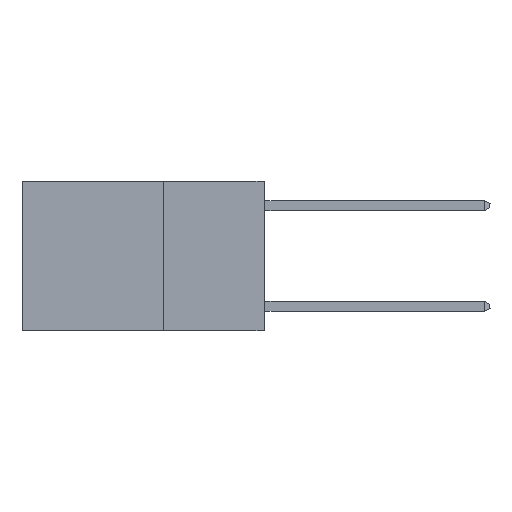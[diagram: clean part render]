
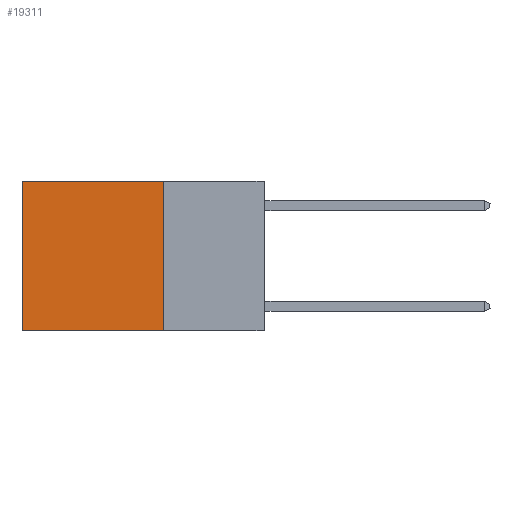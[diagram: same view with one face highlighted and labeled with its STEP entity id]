
A CAD part, left-side view. The second image highlights one B-rep face of the part: STEP entity #19311.
In plain terms, the highlighted planar face has unit normal (-1, 0, 0).
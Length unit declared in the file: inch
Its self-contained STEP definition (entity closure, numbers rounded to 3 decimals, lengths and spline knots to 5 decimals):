
#1014 = LINE ( 'NONE', #16005, #12739 ) ;
#1134 = DIRECTION ( 'NONE',  ( 0., 1., 0. ) ) ;
#2285 = ORIENTED_EDGE ( 'NONE', *, *, #2724, .T. ) ;
#2724 = EDGE_CURVE ( 'NONE', #8821, #21609, #3388, .T. ) ;
#3388 = LINE ( 'NONE', #18354, #5011 ) ;
#3890 = ORIENTED_EDGE ( 'NONE', *, *, #13768, .T. ) ;
#4127 = DIRECTION ( 'NONE',  ( 1., 0., 0. ) ) ;
#4256 = EDGE_LOOP ( 'NONE', ( #3890, #9348, #16654, #2285 ) ) ;
#5011 = VECTOR ( 'NONE', #23999, 39.37008 ) ;
#6788 = CARTESIAN_POINT ( 'NONE',  ( 0.2625, 0.25, -0.37 ) ) ;
#7810 = CARTESIAN_POINT ( 'NONE',  ( 0.2625, 0.25, 0. ) ) ;
#8394 = EDGE_CURVE ( 'NONE', #8821, #18034, #23233, .T. ) ;
#8821 = VERTEX_POINT ( 'NONE', #17912 ) ;
#9348 = ORIENTED_EDGE ( 'NONE', *, *, #21246, .F. ) ;
#9722 = CARTESIAN_POINT ( 'NONE',  ( 0.2625, 0.6, 0. ) ) ;
#10009 = PLANE ( 'NONE',  #22342 ) ;
#11528 = CARTESIAN_POINT ( 'NONE',  ( 0.2625, 0.6, -0.37 ) ) ;
#11941 = DIRECTION ( 'NONE',  ( 0., 0., -1. ) ) ;
#12739 = VECTOR ( 'NONE', #11941, 39.37008 ) ;
#13768 = EDGE_CURVE ( 'NONE', #21609, #14510, #1014, .T. ) ;
#14129 = VECTOR ( 'NONE', #1134, 39.37008 ) ;
#14510 = VERTEX_POINT ( 'NONE', #11528 ) ;
#16004 = DIRECTION ( 'NONE',  ( 0., 0., -1. ) ) ;
#16005 = CARTESIAN_POINT ( 'NONE',  ( 0.2625, 0.6, 0. ) ) ;
#16654 = ORIENTED_EDGE ( 'NONE', *, *, #8394, .F. ) ;
#17506 = DIRECTION ( 'NONE',  ( 0., 0., -1. ) ) ;
#17912 = CARTESIAN_POINT ( 'NONE',  ( 0.2625, 0.25, 0. ) ) ;
#17961 = LINE ( 'NONE', #6788, #14129 ) ;
#18034 = VERTEX_POINT ( 'NONE', #18069 ) ;
#18069 = CARTESIAN_POINT ( 'NONE',  ( 0.2625, 0.25, -0.37 ) ) ;
#18354 = CARTESIAN_POINT ( 'NONE',  ( 0.2625, 0.25, 0. ) ) ;
#19307 = FACE_OUTER_BOUND ( 'NONE', #4256, .T. ) ;
#19311 = ADVANCED_FACE ( 'NONE', ( #19307 ), #10009, .F. ) ;
#19543 = CARTESIAN_POINT ( 'NONE',  ( 0.2625, 0.25, 0. ) ) ;
#21165 = VECTOR ( 'NONE', #16004, 39.37008 ) ;
#21246 = EDGE_CURVE ( 'NONE', #18034, #14510, #17961, .T. ) ;
#21609 = VERTEX_POINT ( 'NONE', #9722 ) ;
#22342 = AXIS2_PLACEMENT_3D ( 'NONE', #7810, #4127, #17506 ) ;
#23233 = LINE ( 'NONE', #19543, #21165 ) ;
#23999 = DIRECTION ( 'NONE',  ( 0., 1., 0. ) ) ;
